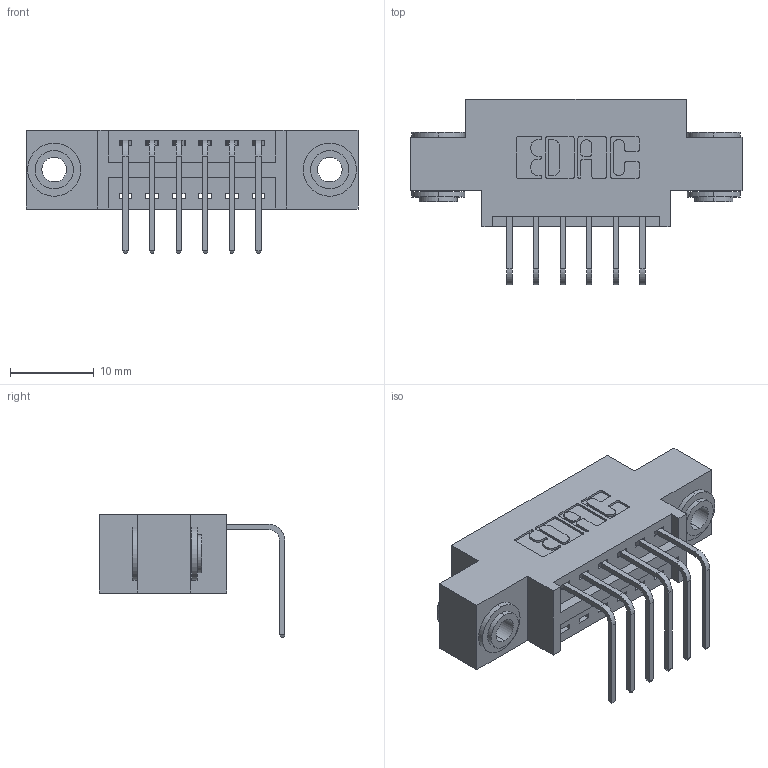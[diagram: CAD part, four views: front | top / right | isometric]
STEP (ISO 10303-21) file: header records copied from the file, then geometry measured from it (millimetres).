
FILE_DESCRIPTION (( 'STEP AP203' ), '1' );
FILE_NAME ('396-006-558-603.STEP', '2018-08-30T23:15:20', ( '' ), ( '' ), 'SwSTEP 2.0', 'SolidWorks 2016', '' );
FILE_SCHEMA (( 'CONFIG_CONTROL_DESIGN' ));
Length unit declared in the file: inch
Products named in the file (4): 346 Part_0.170 Offset - 0.156 Dia-TH; 345-292-001_558 Tail - 2; 345-250-002_345-250-002-102; 396-006-558-603
Assembly tree (9 placements, depth 2):
  396-006-558-603
    346 Part_0.170 Offset - 0.156 Dia-TH
    345-292-001_558 Tail - 2  x6
    345-250-002_345-250-002-102  x2
Bounding box: 39.62 x 22.16 x 14.73 mm (x, y, z)
Volume: 3429.6 mm3; surface area: 4396.9 mm2
Topology: 9 solids, 9 shells, 524 faces, 1509 edges, 994 vertices
Faces by surface type: plane 342, cylinder 174, cone 8
Entity records: 9436 total; most frequent: CARTESIAN_POINT 1609, ORIENTED_EDGE 1542, DIRECTION 1493, EDGE_CURVE 771, VECTOR 591, LINE 591, VERTEX_POINT 510, AXIS2_PLACEMENT_3D 451
